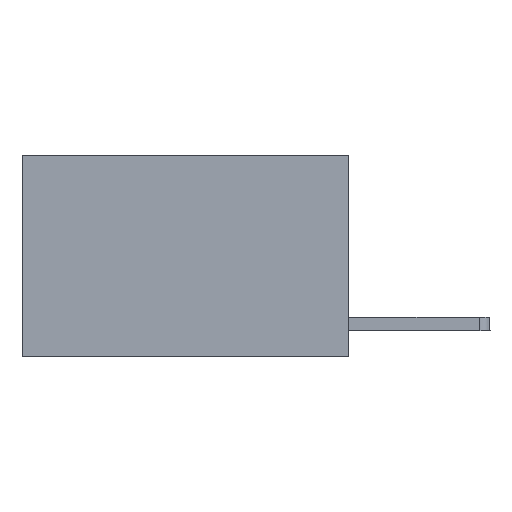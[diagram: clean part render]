
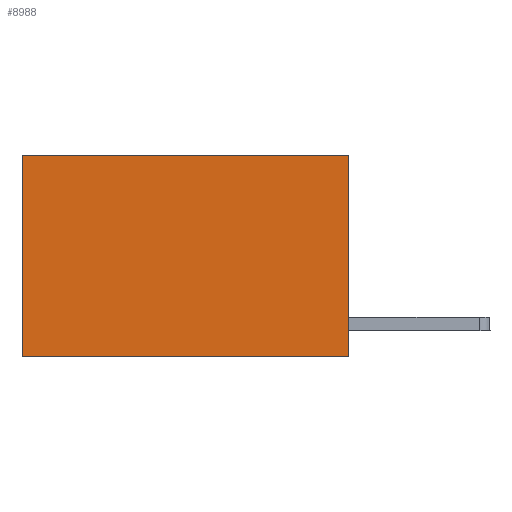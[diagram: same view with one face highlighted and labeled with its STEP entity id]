
A CAD part, left-side view. The second image highlights one B-rep face of the part: STEP entity #8988.
In plain terms, the highlighted planar face has unit normal (-1, 0, 0).
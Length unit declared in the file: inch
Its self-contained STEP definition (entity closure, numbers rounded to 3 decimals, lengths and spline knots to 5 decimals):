
#451 = ORIENTED_EDGE ( 'NONE', *, *, #6806, .T. ) ;
#512 = ORIENTED_EDGE ( 'NONE', *, *, #6965, .T. ) ;
#673 = ORIENTED_EDGE ( 'NONE', *, *, #1704, .F. ) ;
#1011 = DIRECTION ( 'NONE',  ( 0., 0., -1. ) ) ;
#1131 = DIRECTION ( 'NONE',  ( 0., 0., -1. ) ) ;
#1507 = DIRECTION ( 'NONE',  ( 0., 1., 0. ) ) ;
#1704 = EDGE_CURVE ( 'NONE', #8492, #1775, #2409, .T. ) ;
#1775 = VERTEX_POINT ( 'NONE', #1868 ) ;
#1799 = EDGE_LOOP ( 'NONE', ( #451, #4517, #673, #512 ) ) ;
#1868 = CARTESIAN_POINT ( 'NONE',  ( 0.2625, 0., -0.37 ) ) ;
#1976 = CARTESIAN_POINT ( 'NONE',  ( 0.2625, 0., -0.37 ) ) ;
#2046 = CARTESIAN_POINT ( 'NONE',  ( 0.2625, 0.6, -0.37 ) ) ;
#2409 = LINE ( 'NONE', #3987, #8412 ) ;
#2714 = CARTESIAN_POINT ( 'NONE',  ( 0.2625, 0.6, 0. ) ) ;
#2976 = VECTOR ( 'NONE', #1131, 39.37008 ) ;
#3556 = AXIS2_PLACEMENT_3D ( 'NONE', #9378, #4465, #1011 ) ;
#3712 = VECTOR ( 'NONE', #6039, 39.37008 ) ;
#3987 = CARTESIAN_POINT ( 'NONE',  ( 0.2625, 0., 0. ) ) ;
#4154 = FACE_OUTER_BOUND ( 'NONE', #1799, .T. ) ;
#4465 = DIRECTION ( 'NONE',  ( 1., 0., 0. ) ) ;
#4517 = ORIENTED_EDGE ( 'NONE', *, *, #10321, .F. ) ;
#6039 = DIRECTION ( 'NONE',  ( 0., 1., 0. ) ) ;
#6344 = PLANE ( 'NONE',  #3556 ) ;
#6426 = LINE ( 'NONE', #8923, #7986 ) ;
#6806 = EDGE_CURVE ( 'NONE', #8947, #8132, #6968, .T. ) ;
#6965 = EDGE_CURVE ( 'NONE', #8492, #8947, #6426, .T. ) ;
#6968 = LINE ( 'NONE', #2714, #2976 ) ;
#7548 = CARTESIAN_POINT ( 'NONE',  ( 0.2625, 0.6, 0. ) ) ;
#7986 = VECTOR ( 'NONE', #1507, 39.37008 ) ;
#8132 = VERTEX_POINT ( 'NONE', #2046 ) ;
#8412 = VECTOR ( 'NONE', #8792, 39.37008 ) ;
#8492 = VERTEX_POINT ( 'NONE', #9393 ) ;
#8792 = DIRECTION ( 'NONE',  ( 0., 0., -1. ) ) ;
#8923 = CARTESIAN_POINT ( 'NONE',  ( 0.2625, 0., 0. ) ) ;
#8947 = VERTEX_POINT ( 'NONE', #7548 ) ;
#8988 = ADVANCED_FACE ( 'NONE', ( #4154 ), #6344, .F. ) ;
#9378 = CARTESIAN_POINT ( 'NONE',  ( 0.2625, 0., 0. ) ) ;
#9379 = LINE ( 'NONE', #1976, #3712 ) ;
#9393 = CARTESIAN_POINT ( 'NONE',  ( 0.2625, 0., 0. ) ) ;
#10321 = EDGE_CURVE ( 'NONE', #1775, #8132, #9379, .T. ) ;
